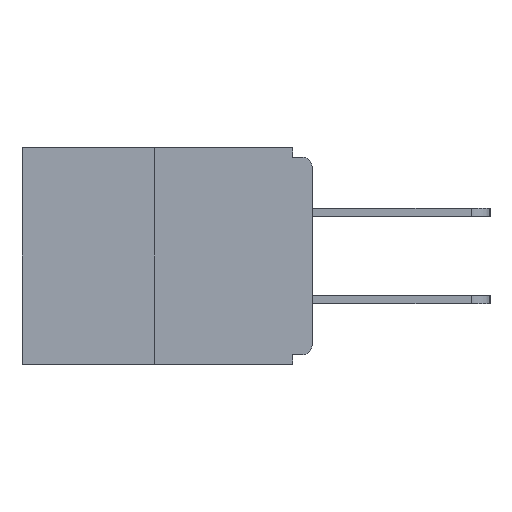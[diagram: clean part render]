
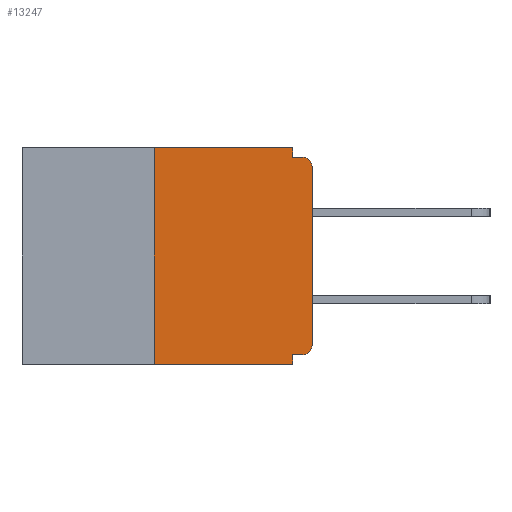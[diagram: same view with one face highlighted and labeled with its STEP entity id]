
A CAD part, left-side view. The second image highlights one B-rep face of the part: STEP entity #13247.
In plain terms, the highlighted planar face has unit normal (-1, 0, 0).
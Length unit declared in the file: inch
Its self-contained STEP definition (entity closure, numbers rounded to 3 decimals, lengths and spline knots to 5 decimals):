
#56 = CARTESIAN_POINT ( 'NONE',  ( 0., 0.031, -0.343 ) ) ;
#490 = VECTOR ( 'NONE', #4622, 39.37008 ) ;
#726 = CARTESIAN_POINT ( 'NONE',  ( 0., 0.015, -0.03 ) ) ;
#910 = EDGE_CURVE ( 'NONE', #9741, #14841, #13048, .T. ) ;
#1602 = ORIENTED_EDGE ( 'NONE', *, *, #16555, .T. ) ;
#1652 = VERTEX_POINT ( 'NONE', #12593 ) ;
#1748 = CARTESIAN_POINT ( 'NONE',  ( 0., 0.25, 0. ) ) ;
#2014 = AXIS2_PLACEMENT_3D ( 'NONE', #726, #30655, #21003 ) ;
#2174 = AXIS2_PLACEMENT_3D ( 'NONE', #16941, #24756, #4519 ) ;
#2288 = EDGE_CURVE ( 'NONE', #1652, #21065, #8918, .T. ) ;
#2301 = EDGE_CURVE ( 'NONE', #14841, #8556, #21433, .T. ) ;
#2334 = VECTOR ( 'NONE', #18950, 39.37008 ) ;
#2351 = ORIENTED_EDGE ( 'NONE', *, *, #910, .T. ) ;
#2381 = LINE ( 'NONE', #12536, #8172 ) ;
#2958 = EDGE_CURVE ( 'NONE', #4986, #19835, #21404, .T. ) ;
#3322 = CARTESIAN_POINT ( 'NONE',  ( 0., 0., -0.03 ) ) ;
#3617 = LINE ( 'NONE', #56, #490 ) ;
#3790 = EDGE_LOOP ( 'NONE', ( #6142, #10654, #9814, #21259, #22172, #2351, #10179, #1602, #24803, #17500 ) ) ;
#4519 = DIRECTION ( 'NONE',  ( 0., 0., -1. ) ) ;
#4622 = DIRECTION ( 'NONE',  ( 0., 0., -1. ) ) ;
#4986 = VERTEX_POINT ( 'NONE', #25681 ) ;
#4996 = LINE ( 'NONE', #1748, #17077 ) ;
#5613 = CIRCLE ( 'NONE', #2014, 0.015 ) ;
#6061 = LINE ( 'NONE', #17971, #27097 ) ;
#6142 = ORIENTED_EDGE ( 'NONE', *, *, #29984, .F. ) ;
#8172 = VECTOR ( 'NONE', #27316, 39.37008 ) ;
#8477 = VECTOR ( 'NONE', #28676, 39.37008 ) ;
#8556 = VERTEX_POINT ( 'NONE', #3322 ) ;
#8880 = CARTESIAN_POINT ( 'NONE',  ( 0., 0., 0. ) ) ;
#8901 = VERTEX_POINT ( 'NONE', #15336 ) ;
#8918 = LINE ( 'NONE', #23492, #2334 ) ;
#8929 = VERTEX_POINT ( 'NONE', #19156 ) ;
#9129 = CARTESIAN_POINT ( 'NONE',  ( 0., 0.015, -0.328 ) ) ;
#9472 = CARTESIAN_POINT ( 'NONE',  ( 0., 0.031, -0.343 ) ) ;
#9739 = VECTOR ( 'NONE', #11525, 39.37008 ) ;
#9741 = VERTEX_POINT ( 'NONE', #9129 ) ;
#9814 = ORIENTED_EDGE ( 'NONE', *, *, #2288, .T. ) ;
#10179 = ORIENTED_EDGE ( 'NONE', *, *, #2301, .T. ) ;
#10654 = ORIENTED_EDGE ( 'NONE', *, *, #19898, .F. ) ;
#11525 = DIRECTION ( 'NONE',  ( 0., 0., 1. ) ) ;
#11751 = DIRECTION ( 'NONE',  ( 1., 0., 0. ) ) ;
#12245 = EDGE_CURVE ( 'NONE', #27133, #4986, #18197, .T. ) ;
#12536 = CARTESIAN_POINT ( 'NONE',  ( 0., 0.46, 0. ) ) ;
#12593 = CARTESIAN_POINT ( 'NONE',  ( 0., 0.25, -0.343 ) ) ;
#13048 = CIRCLE ( 'NONE', #2174, 0.015 ) ;
#13247 = ADVANCED_FACE ( 'NONE', ( #14590 ), #26883, .F. ) ;
#14590 = FACE_OUTER_BOUND ( 'NONE', #3790, .T. ) ;
#14841 = VERTEX_POINT ( 'NONE', #24210 ) ;
#15336 = CARTESIAN_POINT ( 'NONE',  ( 0., 0.25, 0. ) ) ;
#15780 = EDGE_CURVE ( 'NONE', #9741, #8929, #6061, .T. ) ;
#16555 = EDGE_CURVE ( 'NONE', #8556, #19835, #5613, .T. ) ;
#16841 = DIRECTION ( 'NONE',  ( 0., 0., -1. ) ) ;
#16941 = CARTESIAN_POINT ( 'NONE',  ( 0., 0.015, -0.313 ) ) ;
#17077 = VECTOR ( 'NONE', #24134, 39.37008 ) ;
#17500 = ORIENTED_EDGE ( 'NONE', *, *, #12245, .F. ) ;
#17971 = CARTESIAN_POINT ( 'NONE',  ( 0., 0., -0.328 ) ) ;
#18197 = LINE ( 'NONE', #19263, #27513 ) ;
#18548 = CARTESIAN_POINT ( 'NONE',  ( 0., 0.031, 0. ) ) ;
#18694 = CARTESIAN_POINT ( 'NONE',  ( 0., 0., -0.015 ) ) ;
#18950 = DIRECTION ( 'NONE',  ( 0., -1., 0. ) ) ;
#19156 = CARTESIAN_POINT ( 'NONE',  ( 0., 0.031, -0.328 ) ) ;
#19263 = CARTESIAN_POINT ( 'NONE',  ( 0., 0.031, 0. ) ) ;
#19835 = VERTEX_POINT ( 'NONE', #21353 ) ;
#19898 = EDGE_CURVE ( 'NONE', #1652, #8901, #4996, .T. ) ;
#21003 = DIRECTION ( 'NONE',  ( 0., 0., -1. ) ) ;
#21065 = VERTEX_POINT ( 'NONE', #9472 ) ;
#21259 = ORIENTED_EDGE ( 'NONE', *, *, #28322, .F. ) ;
#21353 = CARTESIAN_POINT ( 'NONE',  ( 0., 0.015, -0.015 ) ) ;
#21404 = LINE ( 'NONE', #18694, #8477 ) ;
#21433 = LINE ( 'NONE', #8880, #9739 ) ;
#21567 = CARTESIAN_POINT ( 'NONE',  ( 0., 0.46, 0. ) ) ;
#22172 = ORIENTED_EDGE ( 'NONE', *, *, #15780, .F. ) ;
#23492 = CARTESIAN_POINT ( 'NONE',  ( 0., 0.46, -0.343 ) ) ;
#24134 = DIRECTION ( 'NONE',  ( 0., 0., 1. ) ) ;
#24210 = CARTESIAN_POINT ( 'NONE',  ( 0., 0., -0.313 ) ) ;
#24756 = DIRECTION ( 'NONE',  ( -1., 0., 0. ) ) ;
#24803 = ORIENTED_EDGE ( 'NONE', *, *, #2958, .F. ) ;
#25681 = CARTESIAN_POINT ( 'NONE',  ( 0., 0.031, -0.015 ) ) ;
#26440 = DIRECTION ( 'NONE',  ( 0., 0., -1. ) ) ;
#26883 = PLANE ( 'NONE',  #28601 ) ;
#27097 = VECTOR ( 'NONE', #27853, 39.37008 ) ;
#27133 = VERTEX_POINT ( 'NONE', #18548 ) ;
#27316 = DIRECTION ( 'NONE',  ( 0., -1., 0. ) ) ;
#27513 = VECTOR ( 'NONE', #16841, 39.37008 ) ;
#27853 = DIRECTION ( 'NONE',  ( 0., 1., 0. ) ) ;
#28322 = EDGE_CURVE ( 'NONE', #8929, #21065, #3617, .T. ) ;
#28601 = AXIS2_PLACEMENT_3D ( 'NONE', #21567, #11751, #26440 ) ;
#28676 = DIRECTION ( 'NONE',  ( 0., -1., 0. ) ) ;
#29984 = EDGE_CURVE ( 'NONE', #8901, #27133, #2381, .T. ) ;
#30655 = DIRECTION ( 'NONE',  ( -1., 0., 0. ) ) ;
